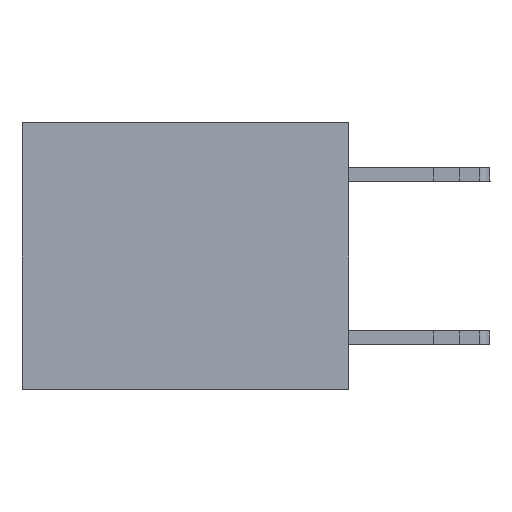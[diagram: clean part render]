
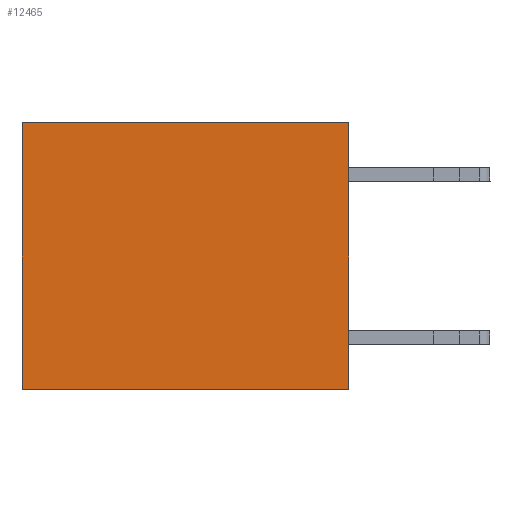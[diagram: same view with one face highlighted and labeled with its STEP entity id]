
A CAD part, left-side view. The second image highlights one B-rep face of the part: STEP entity #12465.
In plain terms, the highlighted planar face has unit normal (-1, 0, 0).
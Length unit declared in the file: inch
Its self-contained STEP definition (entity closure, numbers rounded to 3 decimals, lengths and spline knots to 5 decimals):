
#352 = EDGE_CURVE ( 'NONE', #3506, #19442, #9731, .T. ) ;
#771 = FACE_OUTER_BOUND ( 'NONE', #3272, .T. ) ;
#2662 = VECTOR ( 'NONE', #18104, 39.37008 ) ;
#2690 = VERTEX_POINT ( 'NONE', #11604 ) ;
#3272 = EDGE_LOOP ( 'NONE', ( #19665, #6109, #10061, #4933 ) ) ;
#3506 = VERTEX_POINT ( 'NONE', #5345 ) ;
#3651 = EDGE_CURVE ( 'NONE', #2690, #3506, #21275, .T. ) ;
#3667 = VECTOR ( 'NONE', #10370, 39.37008 ) ;
#3924 = CARTESIAN_POINT ( 'NONE',  ( 0.3165, 0., -0.49 ) ) ;
#3944 = CARTESIAN_POINT ( 'NONE',  ( 0.3165, 0., 0. ) ) ;
#4547 = VECTOR ( 'NONE', #16258, 39.37008 ) ;
#4933 = ORIENTED_EDGE ( 'NONE', *, *, #3651, .T. ) ;
#5345 = CARTESIAN_POINT ( 'NONE',  ( 0.3165, 0.6, 0. ) ) ;
#5460 = DIRECTION ( 'NONE',  ( 1., 0., 0. ) ) ;
#5686 = DIRECTION ( 'NONE',  ( 0., 0., -1. ) ) ;
#6109 = ORIENTED_EDGE ( 'NONE', *, *, #13035, .F. ) ;
#6875 = CARTESIAN_POINT ( 'NONE',  ( 0.3165, 0., -0.49 ) ) ;
#7549 = DIRECTION ( 'NONE',  ( 0., 0., -1. ) ) ;
#8403 = LINE ( 'NONE', #19691, #4547 ) ;
#8895 = VERTEX_POINT ( 'NONE', #20825 ) ;
#9171 = AXIS2_PLACEMENT_3D ( 'NONE', #3924, #5460, #5686 ) ;
#9731 = LINE ( 'NONE', #16277, #17542 ) ;
#10061 = ORIENTED_EDGE ( 'NONE', *, *, #12509, .F. ) ;
#10370 = DIRECTION ( 'NONE',  ( 0., 1., 0. ) ) ;
#11604 = CARTESIAN_POINT ( 'NONE',  ( 0.3165, 0., 0. ) ) ;
#12465 = ADVANCED_FACE ( 'NONE', ( #771 ), #19620, .F. ) ;
#12509 = EDGE_CURVE ( 'NONE', #2690, #8895, #8403, .T. ) ;
#13035 = EDGE_CURVE ( 'NONE', #8895, #19442, #22555, .T. ) ;
#16258 = DIRECTION ( 'NONE',  ( 0., 0., -1. ) ) ;
#16277 = CARTESIAN_POINT ( 'NONE',  ( 0.3165, 0.6, -0.49 ) ) ;
#17542 = VECTOR ( 'NONE', #7549, 39.37008 ) ;
#18104 = DIRECTION ( 'NONE',  ( 0., 1., 0. ) ) ;
#18709 = CARTESIAN_POINT ( 'NONE',  ( 0.3165, 0.6, -0.49 ) ) ;
#19442 = VERTEX_POINT ( 'NONE', #18709 ) ;
#19620 = PLANE ( 'NONE',  #9171 ) ;
#19665 = ORIENTED_EDGE ( 'NONE', *, *, #352, .T. ) ;
#19691 = CARTESIAN_POINT ( 'NONE',  ( 0.3165, 0., -0.49 ) ) ;
#20825 = CARTESIAN_POINT ( 'NONE',  ( 0.3165, 0., -0.49 ) ) ;
#21275 = LINE ( 'NONE', #3944, #2662 ) ;
#22555 = LINE ( 'NONE', #6875, #3667 ) ;
